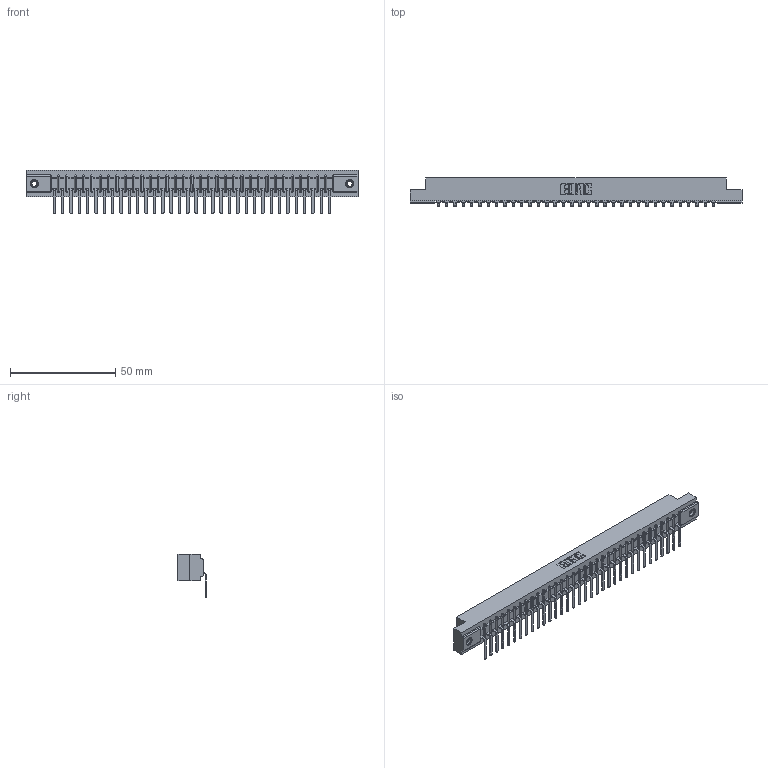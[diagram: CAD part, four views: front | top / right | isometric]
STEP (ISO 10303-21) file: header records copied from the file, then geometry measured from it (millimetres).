
FILE_DESCRIPTION (( 'STEP AP203' ), '1' );
FILE_NAME ('357-034-457-107.STEP', '2020-10-02T11:14:05', ( '' ), ( '' ), 'SwSTEP 2.0', 'SolidWorks 2020', '' );
FILE_SCHEMA (( 'CONFIG_CONTROL_DESIGN' ));
Length unit declared in the file: inch
Products named in the file (4): 307 Part_.156 Dia Mounting Holes; 307-290-002_557; 357-034-457-107; 345-250-001_345-250-005-103
Assembly tree (37 placements, depth 2):
  357-034-457-107
    307 Part_.156 Dia Mounting Holes
    307-290-002_557  x34
    345-250-001_345-250-005-103  x2
Bounding box: 157.73 x 13.32 x 20.66 mm (x, y, z)
Volume: 16898.1 mm3; surface area: 21700.7 mm2
Topology: 37 solids, 37 shells, 2865 faces, 8755 edges, 5734 vertices
Faces by surface type: plane 1700, cylinder 1079, sphere 70, cone 12, torus 4
Entity records: 32173 total; most frequent: CARTESIAN_POINT 5407, ORIENTED_EDGE 5390, DIRECTION 5267, EDGE_CURVE 2695, VECTOR 2059, LINE 2059, VERTEX_POINT 1744, AXIS2_PLACEMENT_3D 1604
